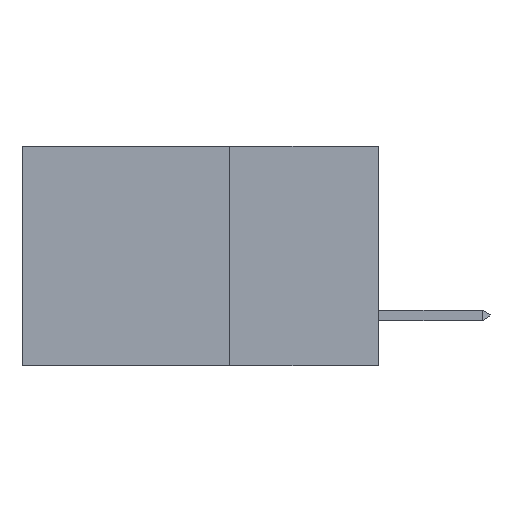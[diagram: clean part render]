
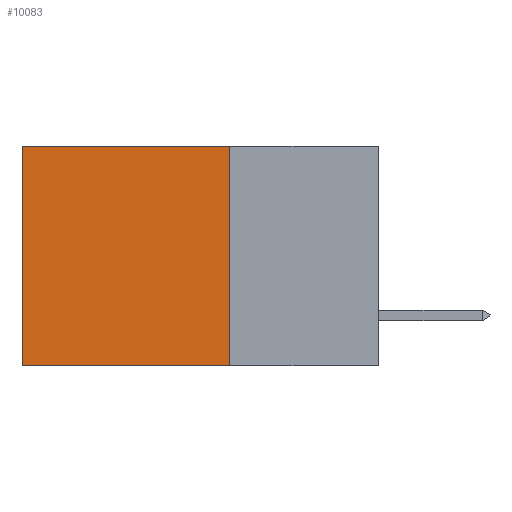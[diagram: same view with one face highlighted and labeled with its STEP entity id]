
A CAD part, left-side view. The second image highlights one B-rep face of the part: STEP entity #10083.
In plain terms, the highlighted planar face has unit normal (-1, 0, 0).
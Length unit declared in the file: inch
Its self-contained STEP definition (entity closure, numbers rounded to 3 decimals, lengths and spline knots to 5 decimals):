
#262 = ORIENTED_EDGE ( 'NONE', *, *, #2347, .T. ) ;
#398 = CARTESIAN_POINT ( 'NONE',  ( 0.2615, 0.25, 0. ) ) ;
#666 = EDGE_LOOP ( 'NONE', ( #16990, #4160, #4647, #262 ) ) ;
#798 = DIRECTION ( 'NONE',  ( 0., 0., -1. ) ) ;
#2347 = EDGE_CURVE ( 'NONE', #14478, #8004, #5437, .T. ) ;
#2614 = LINE ( 'NONE', #18799, #17032 ) ;
#4058 = DIRECTION ( 'NONE',  ( 0., 0., -1. ) ) ;
#4160 = ORIENTED_EDGE ( 'NONE', *, *, #19962, .F. ) ;
#4219 = AXIS2_PLACEMENT_3D ( 'NONE', #9716, #19153, #798 ) ;
#4647 = ORIENTED_EDGE ( 'NONE', *, *, #4844, .F. ) ;
#4844 = EDGE_CURVE ( 'NONE', #14478, #6460, #23854, .T. ) ;
#5073 = VERTEX_POINT ( 'NONE', #11545 ) ;
#5437 = LINE ( 'NONE', #9053, #17520 ) ;
#6394 = CARTESIAN_POINT ( 'NONE',  ( 0.2615, 0.6, 0. ) ) ;
#6460 = VERTEX_POINT ( 'NONE', #12121 ) ;
#7154 = CARTESIAN_POINT ( 'NONE',  ( 0.2615, 0.25, -0.37 ) ) ;
#7909 = FACE_OUTER_BOUND ( 'NONE', #666, .T. ) ;
#8004 = VERTEX_POINT ( 'NONE', #6394 ) ;
#8709 = VECTOR ( 'NONE', #10686, 39.37008 ) ;
#8885 = CARTESIAN_POINT ( 'NONE',  ( 0.2615, 0.25, -0.37 ) ) ;
#9053 = CARTESIAN_POINT ( 'NONE',  ( 0.2615, 0.25, 0. ) ) ;
#9716 = CARTESIAN_POINT ( 'NONE',  ( 0.2615, 0.25, -0.37 ) ) ;
#10083 = ADVANCED_FACE ( 'NONE', ( #7909 ), #11768, .F. ) ;
#10686 = DIRECTION ( 'NONE',  ( 0., 1., 0. ) ) ;
#10857 = DIRECTION ( 'NONE',  ( 0., 1., 0. ) ) ;
#11002 = VECTOR ( 'NONE', #16423, 39.37008 ) ;
#11545 = CARTESIAN_POINT ( 'NONE',  ( 0.2615, 0.6, -0.37 ) ) ;
#11768 = PLANE ( 'NONE',  #4219 ) ;
#12121 = CARTESIAN_POINT ( 'NONE',  ( 0.2615, 0.25, -0.37 ) ) ;
#13559 = EDGE_CURVE ( 'NONE', #8004, #5073, #2614, .T. ) ;
#14478 = VERTEX_POINT ( 'NONE', #398 ) ;
#16423 = DIRECTION ( 'NONE',  ( 0., 0., -1. ) ) ;
#16990 = ORIENTED_EDGE ( 'NONE', *, *, #13559, .T. ) ;
#17032 = VECTOR ( 'NONE', #4058, 39.37008 ) ;
#17520 = VECTOR ( 'NONE', #10857, 39.37008 ) ;
#18799 = CARTESIAN_POINT ( 'NONE',  ( 0.2615, 0.6, -0.37 ) ) ;
#19153 = DIRECTION ( 'NONE',  ( 1., 0., 0. ) ) ;
#19962 = EDGE_CURVE ( 'NONE', #6460, #5073, #23416, .T. ) ;
#23416 = LINE ( 'NONE', #8885, #8709 ) ;
#23854 = LINE ( 'NONE', #7154, #11002 ) ;
